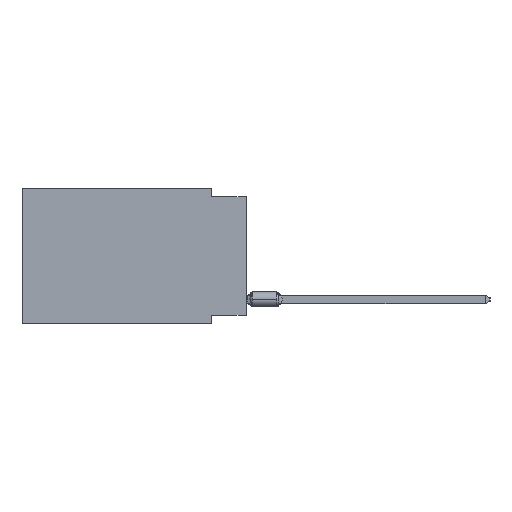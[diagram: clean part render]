
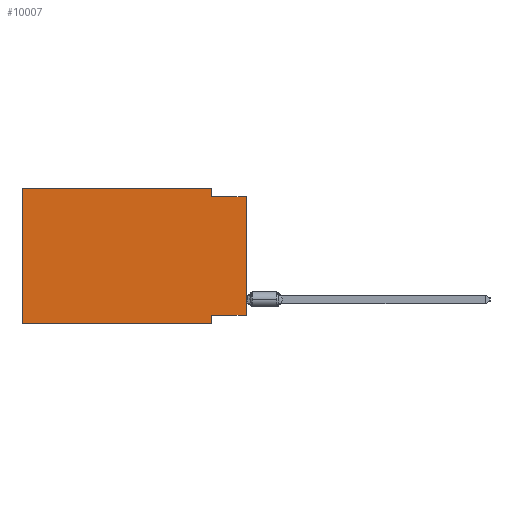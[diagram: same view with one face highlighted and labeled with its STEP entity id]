
A CAD part, left-side view. The second image highlights one B-rep face of the part: STEP entity #10007.
In plain terms, the highlighted planar face has unit normal (-1, 0, 0).
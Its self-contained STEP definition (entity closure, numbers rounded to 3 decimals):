
#13 = VERTEX_POINT ( 'NONE', #12031 ) ;
#291 = LINE ( 'NONE', #27957, #4333 ) ;
#1167 = DIRECTION ( 'NONE',  ( 0., -1., 0. ) ) ;
#1185 = CARTESIAN_POINT ( 'NONE',  ( 0., 2.54, -0.635 ) ) ;
#1230 = LINE ( 'NONE', #13340, #22964 ) ;
#1423 = FACE_OUTER_BOUND ( 'NONE', #13637, .T. ) ;
#1659 = VERTEX_POINT ( 'NONE', #11033 ) ;
#2678 = DIRECTION ( 'NONE',  ( 0., 0., -1. ) ) ;
#2880 = CARTESIAN_POINT ( 'NONE',  ( 0., 0., -9.271 ) ) ;
#3359 = LINE ( 'NONE', #3859, #3496 ) ;
#3496 = VECTOR ( 'NONE', #1167, 1000. ) ;
#3799 = DIRECTION ( 'NONE',  ( 0., 0., -1. ) ) ;
#3859 = CARTESIAN_POINT ( 'NONE',  ( 0., 16.383, 0. ) ) ;
#4240 = EDGE_CURVE ( 'NONE', #13, #16894, #1230, .T. ) ;
#4249 = DIRECTION ( 'NONE',  ( 0., -1., 0. ) ) ;
#4259 = AXIS2_PLACEMENT_3D ( 'NONE', #24356, #11695, #3799 ) ;
#4333 = VECTOR ( 'NONE', #2678, 1000. ) ;
#4427 = CARTESIAN_POINT ( 'NONE',  ( 0., 0., -0.635 ) ) ;
#4833 = DIRECTION ( 'NONE',  ( 0., 0., -1. ) ) ;
#5136 = VERTEX_POINT ( 'NONE', #29734 ) ;
#5870 = VECTOR ( 'NONE', #7860, 1000. ) ;
#6092 = EDGE_CURVE ( 'NONE', #21013, #19543, #22445, .T. ) ;
#6647 = EDGE_CURVE ( 'NONE', #1659, #19543, #20650, .T. ) ;
#7089 = ORIENTED_EDGE ( 'NONE', *, *, #17400, .F. ) ;
#7344 = ORIENTED_EDGE ( 'NONE', *, *, #6647, .T. ) ;
#7860 = DIRECTION ( 'NONE',  ( 0., 0., 1. ) ) ;
#8934 = EDGE_CURVE ( 'NONE', #13, #23214, #24189, .T. ) ;
#10007 = ADVANCED_FACE ( 'NONE', ( #1423 ), #32781, .F. ) ;
#10017 = CARTESIAN_POINT ( 'NONE',  ( 0., 16.383, 0. ) ) ;
#10722 = CARTESIAN_POINT ( 'NONE',  ( 0., 0., -0.635 ) ) ;
#11033 = CARTESIAN_POINT ( 'NONE',  ( 0., 0., -9.271 ) ) ;
#11215 = VECTOR ( 'NONE', #4249, 1000. ) ;
#11229 = ORIENTED_EDGE ( 'NONE', *, *, #25877, .F. ) ;
#11695 = DIRECTION ( 'NONE',  ( 1., 0., 0. ) ) ;
#12031 = CARTESIAN_POINT ( 'NONE',  ( 0., 16.383, -9.906 ) ) ;
#13200 = ORIENTED_EDGE ( 'NONE', *, *, #6092, .F. ) ;
#13340 = CARTESIAN_POINT ( 'NONE',  ( 0., 16.383, 0. ) ) ;
#13637 = EDGE_LOOP ( 'NONE', ( #7344, #13200, #11229, #7089, #22130, #19466, #29743, #26637 ) ) ;
#15339 = DIRECTION ( 'NONE',  ( 0., -1., 0. ) ) ;
#16894 = VERTEX_POINT ( 'NONE', #10017 ) ;
#17400 = EDGE_CURVE ( 'NONE', #16894, #30220, #3359, .T. ) ;
#18364 = LINE ( 'NONE', #2880, #22054 ) ;
#19466 = ORIENTED_EDGE ( 'NONE', *, *, #8934, .T. ) ;
#19543 = VERTEX_POINT ( 'NONE', #10722 ) ;
#19776 = VECTOR ( 'NONE', #15339, 1000. ) ;
#20137 = CARTESIAN_POINT ( 'NONE',  ( 0., 2.54, -9.906 ) ) ;
#20650 = LINE ( 'NONE', #30936, #5870 ) ;
#21013 = VERTEX_POINT ( 'NONE', #1185 ) ;
#22054 = VECTOR ( 'NONE', #31016, 1000. ) ;
#22130 = ORIENTED_EDGE ( 'NONE', *, *, #4240, .F. ) ;
#22445 = LINE ( 'NONE', #4427, #11215 ) ;
#22570 = VECTOR ( 'NONE', #4833, 1000. ) ;
#22938 = CARTESIAN_POINT ( 'NONE',  ( 0., 16.383, -9.906 ) ) ;
#22964 = VECTOR ( 'NONE', #26845, 1000. ) ;
#23214 = VERTEX_POINT ( 'NONE', #20137 ) ;
#24189 = LINE ( 'NONE', #22938, #19776 ) ;
#24356 = CARTESIAN_POINT ( 'NONE',  ( 0., 16.383, 0. ) ) ;
#24548 = EDGE_CURVE ( 'NONE', #5136, #23214, #33143, .T. ) ;
#25492 = EDGE_CURVE ( 'NONE', #1659, #5136, #18364, .T. ) ;
#25877 = EDGE_CURVE ( 'NONE', #30220, #21013, #291, .T. ) ;
#26637 = ORIENTED_EDGE ( 'NONE', *, *, #25492, .F. ) ;
#26845 = DIRECTION ( 'NONE',  ( 0., 0., 1. ) ) ;
#27908 = CARTESIAN_POINT ( 'NONE',  ( 0., 2.54, -9.906 ) ) ;
#27957 = CARTESIAN_POINT ( 'NONE',  ( 0., 2.54, 0. ) ) ;
#29454 = CARTESIAN_POINT ( 'NONE',  ( 0., 2.54, 0. ) ) ;
#29734 = CARTESIAN_POINT ( 'NONE',  ( 0., 2.54, -9.271 ) ) ;
#29743 = ORIENTED_EDGE ( 'NONE', *, *, #24548, .F. ) ;
#30220 = VERTEX_POINT ( 'NONE', #29454 ) ;
#30936 = CARTESIAN_POINT ( 'NONE',  ( 0., 0., 0. ) ) ;
#31016 = DIRECTION ( 'NONE',  ( 0., 1., 0. ) ) ;
#32781 = PLANE ( 'NONE',  #4259 ) ;
#33143 = LINE ( 'NONE', #27908, #22570 ) ;
